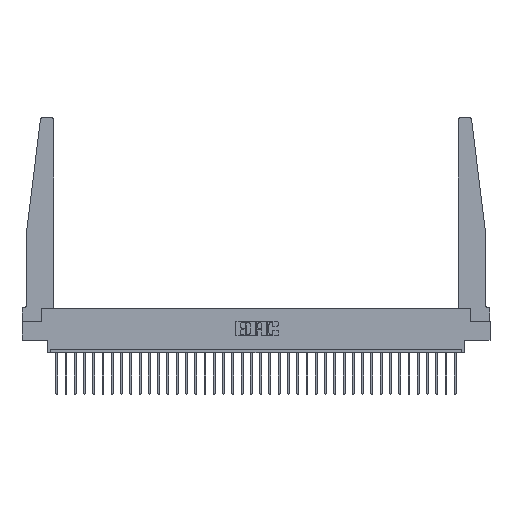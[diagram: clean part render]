
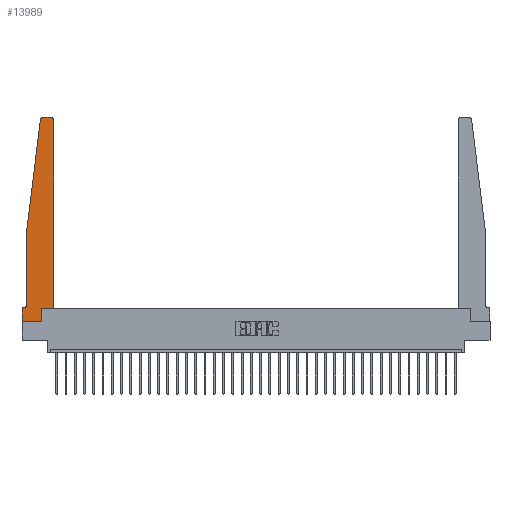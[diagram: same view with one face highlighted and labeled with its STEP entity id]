
A CAD part, top view. The second image highlights one B-rep face of the part: STEP entity #13989.
In plain terms, the highlighted planar face has unit normal (0, 0, 1).
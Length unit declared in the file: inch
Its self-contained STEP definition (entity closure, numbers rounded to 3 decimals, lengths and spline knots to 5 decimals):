
#571 = ORIENTED_EDGE ( 'NONE', *, *, #23345, .T. ) ;
#575 = CARTESIAN_POINT ( 'NONE',  ( 0.015, 0.2375, 0.37 ) ) ;
#1118 = ORIENTED_EDGE ( 'NONE', *, *, #3903, .T. ) ;
#1634 = EDGE_CURVE ( 'NONE', #4341, #17598, #28492, .T. ) ;
#1747 = VERTEX_POINT ( 'NONE', #26865 ) ;
#2319 = DIRECTION ( 'NONE',  ( 0., 1., 0. ) ) ;
#2712 = ORIENTED_EDGE ( 'NONE', *, *, #28171, .T. ) ;
#2787 = CARTESIAN_POINT ( 'NONE',  ( 0.425, 0.18, 0.37 ) ) ;
#3036 = DIRECTION ( 'NONE',  ( -1., 0., 0. ) ) ;
#3211 = CARTESIAN_POINT ( 'NONE',  ( 0.065, 1.25, 0.37 ) ) ;
#3605 = LINE ( 'NONE', #10643, #24846 ) ;
#3903 = EDGE_CURVE ( 'NONE', #4766, #11952, #25278, .T. ) ;
#4013 = AXIS2_PLACEMENT_3D ( 'NONE', #575, #20610, #28078 ) ;
#4053 = LINE ( 'NONE', #2787, #5228 ) ;
#4152 = DIRECTION ( 'NONE',  ( 0., -1., 0. ) ) ;
#4341 = VERTEX_POINT ( 'NONE', #9142 ) ;
#4766 = VERTEX_POINT ( 'NONE', #31732 ) ;
#5227 = ORIENTED_EDGE ( 'NONE', *, *, #28408, .T. ) ;
#5228 = VECTOR ( 'NONE', #7610, 39.37008 ) ;
#5850 = CARTESIAN_POINT ( 'NONE',  ( 0., 0.1875, 0.37 ) ) ;
#7014 = DIRECTION ( 'NONE',  ( 1., 0., 0. ) ) ;
#7247 = CARTESIAN_POINT ( 'NONE',  ( 0.2605, 0., 0.37 ) ) ;
#7277 = CARTESIAN_POINT ( 'NONE',  ( 0.425, 0.18, 0.37 ) ) ;
#7610 = DIRECTION ( 'NONE',  ( 0., 1., 0. ) ) ;
#7741 = CARTESIAN_POINT ( 'NONE',  ( 0.25, 2.75, 0.37 ) ) ;
#7743 = ORIENTED_EDGE ( 'NONE', *, *, #22176, .T. ) ;
#8010 = AXIS2_PLACEMENT_3D ( 'NONE', #9260, #26992, #29348 ) ;
#8064 = ORIENTED_EDGE ( 'NONE', *, *, #24006, .T. ) ;
#8494 = CARTESIAN_POINT ( 'NONE',  ( 0., 0., 0.37 ) ) ;
#8512 = DIRECTION ( 'NONE',  ( -1., 0., 0. ) ) ;
#8646 = DIRECTION ( 'NONE',  ( 1., 0., 0. ) ) ;
#8725 = VECTOR ( 'NONE', #2319, 39.37008 ) ;
#8915 = ORIENTED_EDGE ( 'NONE', *, *, #24917, .T. ) ;
#9142 = CARTESIAN_POINT ( 'NONE',  ( 0.015, 0.1875, 0.37 ) ) ;
#9260 = CARTESIAN_POINT ( 'NONE',  ( 0., 0.1875, 0.37 ) ) ;
#9600 = PLANE ( 'NONE',  #8010 ) ;
#9923 = LINE ( 'NONE', #12668, #8725 ) ;
#10246 = CARTESIAN_POINT ( 'NONE',  ( 0.2605, 0.18, 0.37 ) ) ;
#10505 = CARTESIAN_POINT ( 'NONE',  ( 0.395, 2.72, 0.37 ) ) ;
#10643 = CARTESIAN_POINT ( 'NONE',  ( 0.425, 0.18, 0.37 ) ) ;
#10778 = CARTESIAN_POINT ( 'NONE',  ( 0.395, 2.75, 0.37 ) ) ;
#10909 = CARTESIAN_POINT ( 'NONE',  ( 0.065, 0.1875, 0.37 ) ) ;
#11269 = EDGE_CURVE ( 'NONE', #30644, #17794, #9923, .T. ) ;
#11556 = LINE ( 'NONE', #8494, #13151 ) ;
#11952 = VERTEX_POINT ( 'NONE', #3211 ) ;
#12120 = AXIS2_PLACEMENT_3D ( 'NONE', #10505, #12987, #15456 ) ;
#12155 = CARTESIAN_POINT ( 'NONE',  ( 0., 0., 0.37 ) ) ;
#12668 = CARTESIAN_POINT ( 'NONE',  ( 0.2605, 0.18, 0.37 ) ) ;
#12987 = DIRECTION ( 'NONE',  ( 0., 0., 1. ) ) ;
#13151 = VECTOR ( 'NONE', #28389, 39.37008 ) ;
#13154 = CARTESIAN_POINT ( 'NONE',  ( 0.065, 0.2375, 0.37 ) ) ;
#13989 = ADVANCED_FACE ( 'NONE', ( #19831 ), #9600, .T. ) ;
#14084 = ORIENTED_EDGE ( 'NONE', *, *, #11269, .T. ) ;
#14475 = VECTOR ( 'NONE', #26168, 39.37008 ) ;
#14842 = CARTESIAN_POINT ( 'NONE',  ( 0.065, 1.25, 0.37 ) ) ;
#15456 = DIRECTION ( 'NONE',  ( 1., 0., 0. ) ) ;
#15805 = CARTESIAN_POINT ( 'NONE',  ( 0.27653, 2.75, 0.37 ) ) ;
#16017 = DIRECTION ( 'NONE',  ( 0., 0., 1. ) ) ;
#16463 = CARTESIAN_POINT ( 'NONE',  ( 0.065, 1.25, 0.37 ) ) ;
#17598 = VERTEX_POINT ( 'NONE', #5850 ) ;
#17794 = VERTEX_POINT ( 'NONE', #10246 ) ;
#18104 = LINE ( 'NONE', #7741, #27355 ) ;
#18109 = ORIENTED_EDGE ( 'NONE', *, *, #26546, .T. ) ;
#18711 = VECTOR ( 'NONE', #24241, 39.37008 ) ;
#19827 = EDGE_CURVE ( 'NONE', #30965, #4341, #28114, .T. ) ;
#19831 = FACE_OUTER_BOUND ( 'NONE', #21434, .T. ) ;
#20343 = CIRCLE ( 'NONE', #12120, 0.03 ) ;
#20610 = DIRECTION ( 'NONE',  ( 0., 0., -1. ) ) ;
#21000 = CARTESIAN_POINT ( 'NONE',  ( 0., 0., 0.37 ) ) ;
#21303 = AXIS2_PLACEMENT_3D ( 'NONE', #23876, #16017, #8646 ) ;
#21434 = EDGE_LOOP ( 'NONE', ( #8915, #8064, #1118, #5227, #29162, #27440, #18109, #571, #14084, #2712, #7743, #26844 ) ) ;
#21562 = VERTEX_POINT ( 'NONE', #10778 ) ;
#21848 = LINE ( 'NONE', #21000, #14475 ) ;
#21953 = CIRCLE ( 'NONE', #21303, 0.03 ) ;
#22176 = EDGE_CURVE ( 'NONE', #25551, #1747, #4053, .T. ) ;
#22874 = LINE ( 'NONE', #16463, #31763 ) ;
#23345 = EDGE_CURVE ( 'NONE', #24574, #30644, #11556, .T. ) ;
#23876 = CARTESIAN_POINT ( 'NONE',  ( 0.27653, 2.72, 0.37 ) ) ;
#24006 = EDGE_CURVE ( 'NONE', #30702, #4766, #21953, .T. ) ;
#24241 = DIRECTION ( 'NONE',  ( -0.122, -0.992, 0. ) ) ;
#24574 = VERTEX_POINT ( 'NONE', #12155 ) ;
#24846 = VECTOR ( 'NONE', #7014, 39.37008 ) ;
#24917 = EDGE_CURVE ( 'NONE', #21562, #30702, #18104, .T. ) ;
#25278 = LINE ( 'NONE', #14842, #18711 ) ;
#25405 = VECTOR ( 'NONE', #8512, 39.37008 ) ;
#25551 = VERTEX_POINT ( 'NONE', #7277 ) ;
#26168 = DIRECTION ( 'NONE',  ( 0., -1., 0. ) ) ;
#26546 = EDGE_CURVE ( 'NONE', #17598, #24574, #21848, .T. ) ;
#26844 = ORIENTED_EDGE ( 'NONE', *, *, #31521, .T. ) ;
#26865 = CARTESIAN_POINT ( 'NONE',  ( 0.425, 2.72, 0.37 ) ) ;
#26992 = DIRECTION ( 'NONE',  ( 0., 0., 1. ) ) ;
#27355 = VECTOR ( 'NONE', #3036, 39.37008 ) ;
#27440 = ORIENTED_EDGE ( 'NONE', *, *, #1634, .T. ) ;
#28078 = DIRECTION ( 'NONE',  ( -1., 0., 0. ) ) ;
#28114 = CIRCLE ( 'NONE', #4013, 0.05 ) ;
#28171 = EDGE_CURVE ( 'NONE', #17794, #25551, #3605, .T. ) ;
#28389 = DIRECTION ( 'NONE',  ( 1., 0., 0. ) ) ;
#28408 = EDGE_CURVE ( 'NONE', #11952, #30965, #22874, .T. ) ;
#28492 = LINE ( 'NONE', #10909, #25405 ) ;
#29162 = ORIENTED_EDGE ( 'NONE', *, *, #19827, .T. ) ;
#29348 = DIRECTION ( 'NONE',  ( 1., 0., 0. ) ) ;
#30644 = VERTEX_POINT ( 'NONE', #7247 ) ;
#30702 = VERTEX_POINT ( 'NONE', #15805 ) ;
#30965 = VERTEX_POINT ( 'NONE', #13154 ) ;
#31521 = EDGE_CURVE ( 'NONE', #1747, #21562, #20343, .T. ) ;
#31732 = CARTESIAN_POINT ( 'NONE',  ( 0.24675, 2.72367, 0.37 ) ) ;
#31763 = VECTOR ( 'NONE', #4152, 39.37008 ) ;
